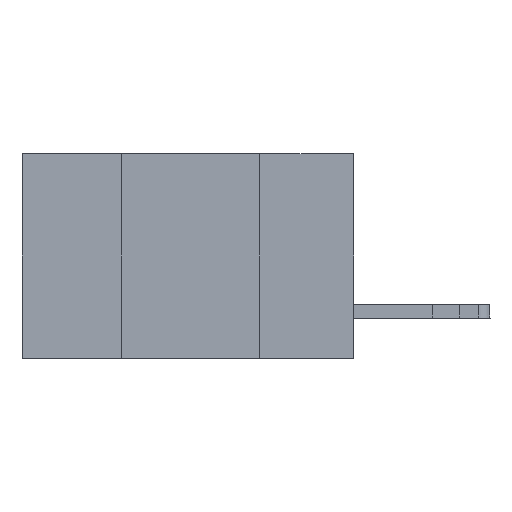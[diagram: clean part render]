
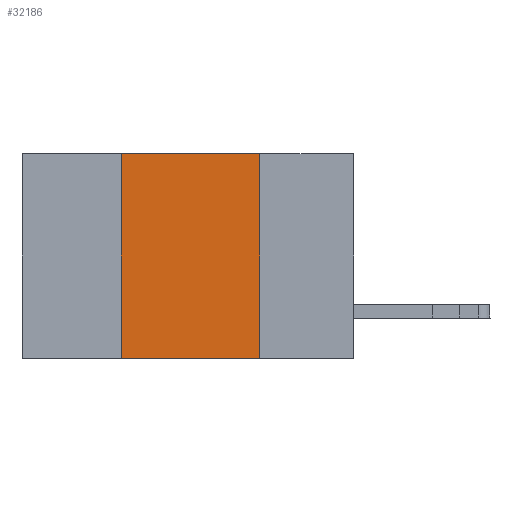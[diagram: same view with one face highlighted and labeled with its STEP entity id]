
A CAD part, left-side view. The second image highlights one B-rep face of the part: STEP entity #32186.
In plain terms, the highlighted planar face has unit normal (-1, 0, 0).
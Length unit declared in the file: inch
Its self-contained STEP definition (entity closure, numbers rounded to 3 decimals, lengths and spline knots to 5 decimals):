
#218 = DIRECTION ( 'NONE',  ( 0., 0., 1. ) ) ;
#4473 = CARTESIAN_POINT ( 'NONE',  ( 0., 0.17, 0. ) ) ;
#6254 = CARTESIAN_POINT ( 'NONE',  ( 0., 0.42, 0. ) ) ;
#8577 = EDGE_CURVE ( 'NONE', #25207, #22712, #12725, .T. ) ;
#8796 = ORIENTED_EDGE ( 'NONE', *, *, #8577, .F. ) ;
#8863 = EDGE_CURVE ( 'NONE', #20292, #25207, #23779, .T. ) ;
#10569 = ORIENTED_EDGE ( 'NONE', *, *, #8863, .F. ) ;
#12134 = DIRECTION ( 'NONE',  ( 1., 0., 0. ) ) ;
#12685 = CARTESIAN_POINT ( 'NONE',  ( 0., 0.17, -0.37 ) ) ;
#12725 = LINE ( 'NONE', #18010, #37220 ) ;
#13763 = EDGE_LOOP ( 'NONE', ( #15257, #8796, #10569, #35977 ) ) ;
#15257 = ORIENTED_EDGE ( 'NONE', *, *, #33124, .F. ) ;
#15960 = DIRECTION ( 'NONE',  ( 0., 0., -1. ) ) ;
#16973 = DIRECTION ( 'NONE',  ( 0., -1., 0. ) ) ;
#17790 = EDGE_CURVE ( 'NONE', #20292, #21833, #28491, .T. ) ;
#18010 = CARTESIAN_POINT ( 'NONE',  ( 0., 0.6, 0. ) ) ;
#18057 = VECTOR ( 'NONE', #15960, 39.37008 ) ;
#18619 = VECTOR ( 'NONE', #218, 39.37008 ) ;
#18794 = LINE ( 'NONE', #4473, #18057 ) ;
#20292 = VERTEX_POINT ( 'NONE', #25543 ) ;
#20829 = DIRECTION ( 'NONE',  ( 0., 0., -1. ) ) ;
#21013 = CARTESIAN_POINT ( 'NONE',  ( 0., 0.6, 0. ) ) ;
#21833 = VERTEX_POINT ( 'NONE', #12685 ) ;
#22712 = VERTEX_POINT ( 'NONE', #32357 ) ;
#23681 = DIRECTION ( 'NONE',  ( 0., -1., 0. ) ) ;
#23779 = LINE ( 'NONE', #6254, #18619 ) ;
#23792 = VECTOR ( 'NONE', #16973, 39.37008 ) ;
#25207 = VERTEX_POINT ( 'NONE', #26953 ) ;
#25543 = CARTESIAN_POINT ( 'NONE',  ( 0., 0.42, -0.37 ) ) ;
#26671 = FACE_OUTER_BOUND ( 'NONE', #13763, .T. ) ;
#26953 = CARTESIAN_POINT ( 'NONE',  ( 0., 0.42, 0. ) ) ;
#27044 = PLANE ( 'NONE',  #33135 ) ;
#28491 = LINE ( 'NONE', #34859, #23792 ) ;
#32186 = ADVANCED_FACE ( 'NONE', ( #26671 ), #27044, .F. ) ;
#32357 = CARTESIAN_POINT ( 'NONE',  ( 0., 0.17, 0. ) ) ;
#33124 = EDGE_CURVE ( 'NONE', #22712, #21833, #18794, .T. ) ;
#33135 = AXIS2_PLACEMENT_3D ( 'NONE', #21013, #12134, #20829 ) ;
#34859 = CARTESIAN_POINT ( 'NONE',  ( 0., 0.6, -0.37 ) ) ;
#35977 = ORIENTED_EDGE ( 'NONE', *, *, #17790, .T. ) ;
#37220 = VECTOR ( 'NONE', #23681, 39.37008 ) ;
